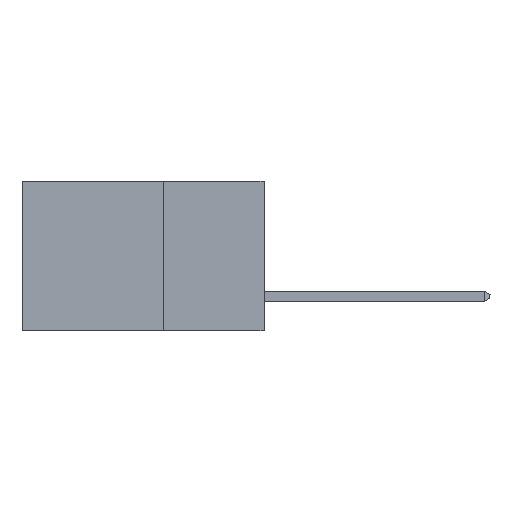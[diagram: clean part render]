
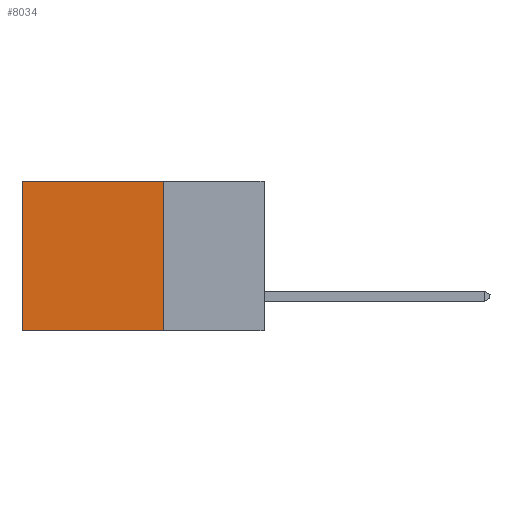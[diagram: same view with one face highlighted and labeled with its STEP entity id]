
A CAD part, left-side view. The second image highlights one B-rep face of the part: STEP entity #8034.
In plain terms, the highlighted planar face has unit normal (-1, 0, 0).
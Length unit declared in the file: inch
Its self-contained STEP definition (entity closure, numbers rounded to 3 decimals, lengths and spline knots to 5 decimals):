
#153 = CARTESIAN_POINT ( 'NONE',  ( 0.2615, 0.25, -0.37 ) ) ;
#193 = EDGE_LOOP ( 'NONE', ( #11118, #1574, #15498, #3010 ) ) ;
#442 = CARTESIAN_POINT ( 'NONE',  ( 0.2615, 0.6, -0.37 ) ) ;
#870 = EDGE_CURVE ( 'NONE', #4767, #1923, #15740, .T. ) ;
#1534 = CARTESIAN_POINT ( 'NONE',  ( 0.2615, 0.25, -0.37 ) ) ;
#1574 = ORIENTED_EDGE ( 'NONE', *, *, #11300, .F. ) ;
#1823 = CARTESIAN_POINT ( 'NONE',  ( 0.2615, 0.25, -0.37 ) ) ;
#1906 = DIRECTION ( 'NONE',  ( 0., 0., -1. ) ) ;
#1923 = VERTEX_POINT ( 'NONE', #4750 ) ;
#2537 = DIRECTION ( 'NONE',  ( 1., 0., 0. ) ) ;
#2622 = PLANE ( 'NONE',  #6647 ) ;
#2857 = VECTOR ( 'NONE', #1906, 39.37008 ) ;
#3010 = ORIENTED_EDGE ( 'NONE', *, *, #14807, .T. ) ;
#3870 = EDGE_CURVE ( 'NONE', #17799, #9058, #11455, .T. ) ;
#4750 = CARTESIAN_POINT ( 'NONE',  ( 0.2615, 0.6, -0.37 ) ) ;
#4767 = VERTEX_POINT ( 'NONE', #5917 ) ;
#4974 = VECTOR ( 'NONE', #5526, 39.37008 ) ;
#5491 = LINE ( 'NONE', #15422, #8506 ) ;
#5526 = DIRECTION ( 'NONE',  ( 0., 1., 0. ) ) ;
#5917 = CARTESIAN_POINT ( 'NONE',  ( 0.2615, 0.6, 0. ) ) ;
#6647 = AXIS2_PLACEMENT_3D ( 'NONE', #10811, #2537, #16459 ) ;
#8034 = ADVANCED_FACE ( 'NONE', ( #9801 ), #2622, .F. ) ;
#8506 = VECTOR ( 'NONE', #15158, 39.37008 ) ;
#9058 = VERTEX_POINT ( 'NONE', #1823 ) ;
#9801 = FACE_OUTER_BOUND ( 'NONE', #193, .T. ) ;
#10288 = CARTESIAN_POINT ( 'NONE',  ( 0.2615, 0.25, 0. ) ) ;
#10811 = CARTESIAN_POINT ( 'NONE',  ( 0.2615, 0.25, -0.37 ) ) ;
#11118 = ORIENTED_EDGE ( 'NONE', *, *, #870, .T. ) ;
#11300 = EDGE_CURVE ( 'NONE', #9058, #1923, #13838, .T. ) ;
#11455 = LINE ( 'NONE', #1534, #14389 ) ;
#12648 = DIRECTION ( 'NONE',  ( 0., 0., -1. ) ) ;
#13838 = LINE ( 'NONE', #153, #4974 ) ;
#14389 = VECTOR ( 'NONE', #12648, 39.37008 ) ;
#14807 = EDGE_CURVE ( 'NONE', #17799, #4767, #5491, .T. ) ;
#15158 = DIRECTION ( 'NONE',  ( 0., 1., 0. ) ) ;
#15422 = CARTESIAN_POINT ( 'NONE',  ( 0.2615, 0.25, 0. ) ) ;
#15498 = ORIENTED_EDGE ( 'NONE', *, *, #3870, .F. ) ;
#15740 = LINE ( 'NONE', #442, #2857 ) ;
#16459 = DIRECTION ( 'NONE',  ( 0., 0., -1. ) ) ;
#17799 = VERTEX_POINT ( 'NONE', #10288 ) ;
